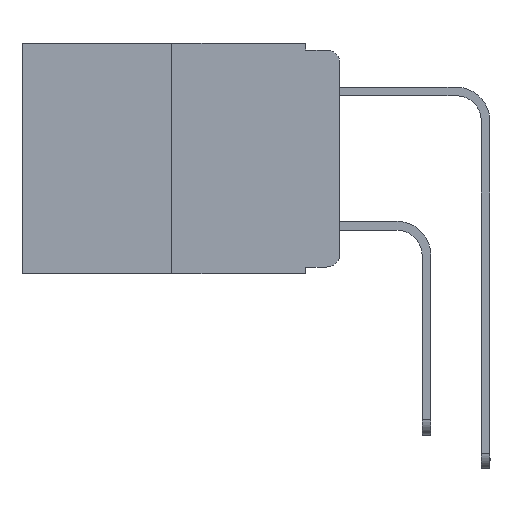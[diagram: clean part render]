
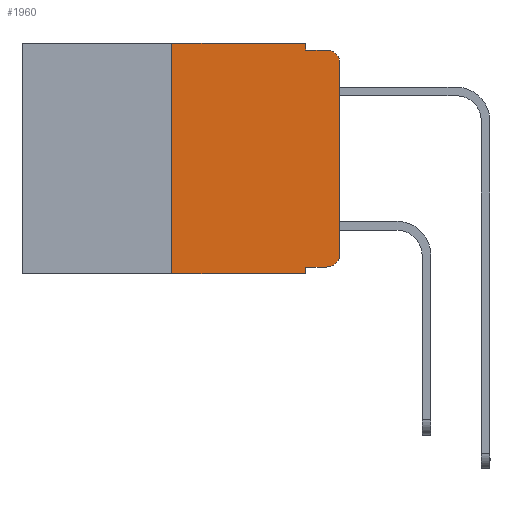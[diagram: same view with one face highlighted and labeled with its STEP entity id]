
A CAD part, left-side view. The second image highlights one B-rep face of the part: STEP entity #1960.
In plain terms, the highlighted planar face has unit normal (-1, 0, 0).
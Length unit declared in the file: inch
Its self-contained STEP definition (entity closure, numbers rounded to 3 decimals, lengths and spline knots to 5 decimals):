
#28 = VERTEX_POINT ( 'NONE', #3407 ) ;
#40 = EDGE_CURVE ( 'NONE', #7876, #10500, #10294, .T. ) ;
#133 = DIRECTION ( 'NONE',  ( 0., 0., -1. ) ) ;
#198 = ORIENTED_EDGE ( 'NONE', *, *, #2876, .F. ) ;
#297 = ORIENTED_EDGE ( 'NONE', *, *, #3672, .T. ) ;
#451 = EDGE_LOOP ( 'NONE', ( #7753, #4925, #1688, #11698, #5810, #4330, #884, #198, #8744, #297 ) ) ;
#462 = AXIS2_PLACEMENT_3D ( 'NONE', #5412, #9350, #11227 ) ;
#670 = VECTOR ( 'NONE', #5596, 39.37008 ) ;
#884 = ORIENTED_EDGE ( 'NONE', *, *, #9285, .T. ) ;
#899 = VERTEX_POINT ( 'NONE', #2695 ) ;
#1006 = VERTEX_POINT ( 'NONE', #1441 ) ;
#1323 = CARTESIAN_POINT ( 'NONE',  ( 0., 0.02, -0.333 ) ) ;
#1420 = CARTESIAN_POINT ( 'NONE',  ( 0., 0.051, 0. ) ) ;
#1441 = CARTESIAN_POINT ( 'NONE',  ( 0., 0., -0.313 ) ) ;
#1457 = DIRECTION ( 'NONE',  ( 0., 0., 1. ) ) ;
#1688 = ORIENTED_EDGE ( 'NONE', *, *, #4708, .F. ) ;
#1757 = VECTOR ( 'NONE', #5299, 39.37008 ) ;
#1788 = CARTESIAN_POINT ( 'NONE',  ( 0., 0.25, 0. ) ) ;
#1881 = CARTESIAN_POINT ( 'NONE',  ( 0., 0., -0.03 ) ) ;
#1939 = DIRECTION ( 'NONE',  ( 0., -1., 0. ) ) ;
#1949 = DIRECTION ( 'NONE',  ( 0., 0., -1. ) ) ;
#1960 = ADVANCED_FACE ( 'NONE', ( #3631 ), #7691, .F. ) ;
#2020 = VECTOR ( 'NONE', #1457, 39.37008 ) ;
#2055 = CARTESIAN_POINT ( 'NONE',  ( 0., 0.051, 0. ) ) ;
#2226 = DIRECTION ( 'NONE',  ( 0., -1., 0. ) ) ;
#2277 = LINE ( 'NONE', #7180, #1757 ) ;
#2432 = VERTEX_POINT ( 'NONE', #1323 ) ;
#2648 = CARTESIAN_POINT ( 'NONE',  ( 0., 0.051, -0.333 ) ) ;
#2695 = CARTESIAN_POINT ( 'NONE',  ( 0., 0.051, -0.01 ) ) ;
#2849 = DIRECTION ( 'NONE',  ( -1., 0., 0. ) ) ;
#2876 = EDGE_CURVE ( 'NONE', #8173, #28, #8849, .T. ) ;
#2999 = CARTESIAN_POINT ( 'NONE',  ( 0., 0.051, 0. ) ) ;
#3123 = VECTOR ( 'NONE', #133, 39.37008 ) ;
#3316 = DIRECTION ( 'NONE',  ( 0., -1., 0. ) ) ;
#3407 = CARTESIAN_POINT ( 'NONE',  ( 0., 0.051, -0.343 ) ) ;
#3497 = CIRCLE ( 'NONE', #7304, 0.02 ) ;
#3631 = FACE_OUTER_BOUND ( 'NONE', #451, .T. ) ;
#3672 = EDGE_CURVE ( 'NONE', #2432, #1006, #3497, .T. ) ;
#3811 = VECTOR ( 'NONE', #3316, 39.37008 ) ;
#3892 = DIRECTION ( 'NONE',  ( 1., 0., 0. ) ) ;
#3923 = LINE ( 'NONE', #2055, #6366 ) ;
#4014 = EDGE_CURVE ( 'NONE', #6886, #899, #3923, .T. ) ;
#4330 = ORIENTED_EDGE ( 'NONE', *, *, #40, .F. ) ;
#4708 = EDGE_CURVE ( 'NONE', #899, #7254, #11064, .T. ) ;
#4720 = DIRECTION ( 'NONE',  ( 0., 0., -1. ) ) ;
#4925 = ORIENTED_EDGE ( 'NONE', *, *, #12129, .T. ) ;
#5299 = DIRECTION ( 'NONE',  ( 0., -1., 0. ) ) ;
#5412 = CARTESIAN_POINT ( 'NONE',  ( 0., 0.02, -0.03 ) ) ;
#5596 = DIRECTION ( 'NONE',  ( 0., 0., 1. ) ) ;
#5810 = ORIENTED_EDGE ( 'NONE', *, *, #9357, .F. ) ;
#6029 = VECTOR ( 'NONE', #1939, 39.37008 ) ;
#6150 = CARTESIAN_POINT ( 'NONE',  ( 0., 0.473, 0. ) ) ;
#6366 = VECTOR ( 'NONE', #6709, 39.37008 ) ;
#6554 = VERTEX_POINT ( 'NONE', #1881 ) ;
#6709 = DIRECTION ( 'NONE',  ( 0., 0., -1. ) ) ;
#6886 = VERTEX_POINT ( 'NONE', #1420 ) ;
#7180 = CARTESIAN_POINT ( 'NONE',  ( 0., 0.473, -0.343 ) ) ;
#7254 = VERTEX_POINT ( 'NONE', #8355 ) ;
#7304 = AXIS2_PLACEMENT_3D ( 'NONE', #9939, #2849, #1949 ) ;
#7333 = CARTESIAN_POINT ( 'NONE',  ( 0., 0.25, 0. ) ) ;
#7606 = LINE ( 'NONE', #12634, #670 ) ;
#7691 = PLANE ( 'NONE',  #12207 ) ;
#7753 = ORIENTED_EDGE ( 'NONE', *, *, #12215, .T. ) ;
#7876 = VERTEX_POINT ( 'NONE', #12535 ) ;
#8026 = CARTESIAN_POINT ( 'NONE',  ( 0., 0.051, -0.01 ) ) ;
#8173 = VERTEX_POINT ( 'NONE', #2648 ) ;
#8355 = CARTESIAN_POINT ( 'NONE',  ( 0., 0.02, -0.01 ) ) ;
#8744 = ORIENTED_EDGE ( 'NONE', *, *, #12399, .T. ) ;
#8849 = LINE ( 'NONE', #2999, #3123 ) ;
#9112 = CIRCLE ( 'NONE', #462, 0.02 ) ;
#9285 = EDGE_CURVE ( 'NONE', #7876, #28, #2277, .T. ) ;
#9350 = DIRECTION ( 'NONE',  ( -1., 0., 0. ) ) ;
#9357 = EDGE_CURVE ( 'NONE', #10500, #6886, #11060, .T. ) ;
#9939 = CARTESIAN_POINT ( 'NONE',  ( 0., 0.02, -0.313 ) ) ;
#10294 = LINE ( 'NONE', #7333, #2020 ) ;
#10500 = VERTEX_POINT ( 'NONE', #1788 ) ;
#10772 = LINE ( 'NONE', #10965, #6029 ) ;
#10965 = CARTESIAN_POINT ( 'NONE',  ( 0., 0.051, -0.333 ) ) ;
#10983 = VECTOR ( 'NONE', #2226, 39.37008 ) ;
#11060 = LINE ( 'NONE', #6150, #3811 ) ;
#11064 = LINE ( 'NONE', #8026, #10983 ) ;
#11227 = DIRECTION ( 'NONE',  ( 0., 0., -1. ) ) ;
#11500 = CARTESIAN_POINT ( 'NONE',  ( 0., 0.473, 0. ) ) ;
#11698 = ORIENTED_EDGE ( 'NONE', *, *, #4014, .F. ) ;
#12129 = EDGE_CURVE ( 'NONE', #6554, #7254, #9112, .T. ) ;
#12207 = AXIS2_PLACEMENT_3D ( 'NONE', #11500, #3892, #4720 ) ;
#12215 = EDGE_CURVE ( 'NONE', #1006, #6554, #7606, .T. ) ;
#12399 = EDGE_CURVE ( 'NONE', #8173, #2432, #10772, .T. ) ;
#12535 = CARTESIAN_POINT ( 'NONE',  ( 0., 0.25, -0.343 ) ) ;
#12634 = CARTESIAN_POINT ( 'NONE',  ( 0., 0., 0. ) ) ;
